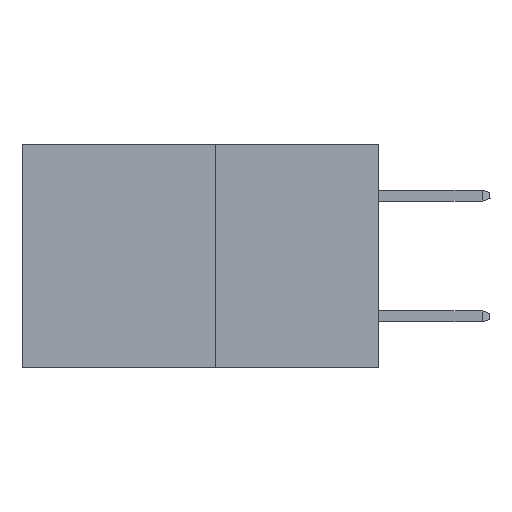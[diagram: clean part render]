
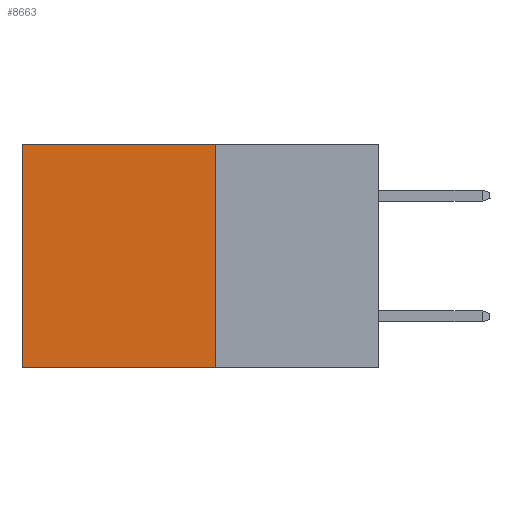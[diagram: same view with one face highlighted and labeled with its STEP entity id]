
A CAD part, left-side view. The second image highlights one B-rep face of the part: STEP entity #8663.
In plain terms, the highlighted planar face has unit normal (-1, 0, 0).
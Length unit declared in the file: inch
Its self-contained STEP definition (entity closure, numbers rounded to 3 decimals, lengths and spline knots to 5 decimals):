
#181 = LINE ( 'NONE', #303, #11334 ) ;
#303 = CARTESIAN_POINT ( 'NONE',  ( 0.277, 0.59, -0.37 ) ) ;
#742 = EDGE_CURVE ( 'NONE', #5803, #17837, #14770, .T. ) ;
#1126 = ORIENTED_EDGE ( 'NONE', *, *, #10406, .T. ) ;
#1504 = CARTESIAN_POINT ( 'NONE',  ( 0.277, 0.27, 0. ) ) ;
#1905 = ORIENTED_EDGE ( 'NONE', *, *, #10242, .T. ) ;
#2054 = VERTEX_POINT ( 'NONE', #3165 ) ;
#2416 = ORIENTED_EDGE ( 'NONE', *, *, #742, .F. ) ;
#2497 = EDGE_LOOP ( 'NONE', ( #1126, #10049, #2416, #1905 ) ) ;
#2531 = VERTEX_POINT ( 'NONE', #13434 ) ;
#2891 = AXIS2_PLACEMENT_3D ( 'NONE', #5265, #16603, #8158 ) ;
#3165 = CARTESIAN_POINT ( 'NONE',  ( 0.277, 0.59, 0. ) ) ;
#4394 = DIRECTION ( 'NONE',  ( 0., 1., 0. ) ) ;
#5265 = CARTESIAN_POINT ( 'NONE',  ( 0.277, 0.27, -0.37 ) ) ;
#5803 = VERTEX_POINT ( 'NONE', #14512 ) ;
#6839 = VECTOR ( 'NONE', #4394, 39.37008 ) ;
#8158 = DIRECTION ( 'NONE',  ( 0., 0., -1. ) ) ;
#8454 = VECTOR ( 'NONE', #13811, 39.37008 ) ;
#8663 = ADVANCED_FACE ( 'NONE', ( #15228 ), #15207, .F. ) ;
#9455 = DIRECTION ( 'NONE',  ( 0., 0., -1. ) ) ;
#9493 = LINE ( 'NONE', #1504, #6839 ) ;
#10049 = ORIENTED_EDGE ( 'NONE', *, *, #15717, .F. ) ;
#10242 = EDGE_CURVE ( 'NONE', #5803, #2054, #9493, .T. ) ;
#10406 = EDGE_CURVE ( 'NONE', #2054, #2531, #181, .T. ) ;
#10489 = CARTESIAN_POINT ( 'NONE',  ( 0.277, 0.27, -0.37 ) ) ;
#11334 = VECTOR ( 'NONE', #16129, 39.37008 ) ;
#13434 = CARTESIAN_POINT ( 'NONE',  ( 0.277, 0.59, -0.37 ) ) ;
#13811 = DIRECTION ( 'NONE',  ( 0., 1., 0. ) ) ;
#14512 = CARTESIAN_POINT ( 'NONE',  ( 0.277, 0.27, 0. ) ) ;
#14770 = LINE ( 'NONE', #16419, #17953 ) ;
#15207 = PLANE ( 'NONE',  #2891 ) ;
#15228 = FACE_OUTER_BOUND ( 'NONE', #2497, .T. ) ;
#15717 = EDGE_CURVE ( 'NONE', #17837, #2531, #18254, .T. ) ;
#16129 = DIRECTION ( 'NONE',  ( 0., 0., -1. ) ) ;
#16419 = CARTESIAN_POINT ( 'NONE',  ( 0.277, 0.27, -0.37 ) ) ;
#16603 = DIRECTION ( 'NONE',  ( 1., 0., 0. ) ) ;
#17837 = VERTEX_POINT ( 'NONE', #10489 ) ;
#17875 = CARTESIAN_POINT ( 'NONE',  ( 0.277, 0.27, -0.37 ) ) ;
#17953 = VECTOR ( 'NONE', #9455, 39.37008 ) ;
#18254 = LINE ( 'NONE', #17875, #8454 ) ;
